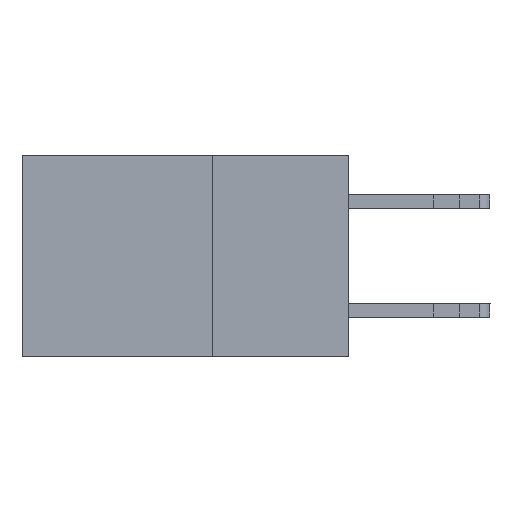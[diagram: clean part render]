
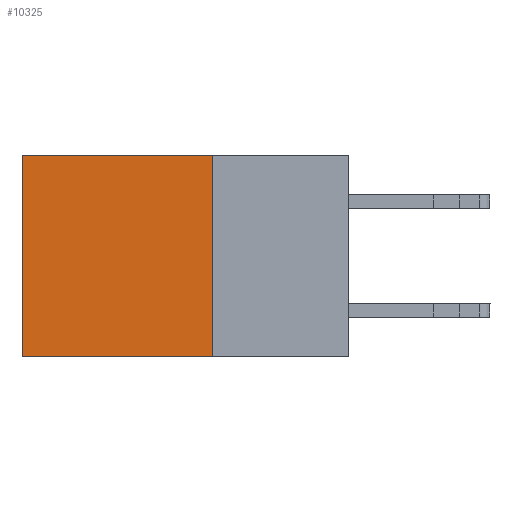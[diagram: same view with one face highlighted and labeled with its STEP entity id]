
A CAD part, left-side view. The second image highlights one B-rep face of the part: STEP entity #10325.
In plain terms, the highlighted planar face has unit normal (-1, 0, 0).
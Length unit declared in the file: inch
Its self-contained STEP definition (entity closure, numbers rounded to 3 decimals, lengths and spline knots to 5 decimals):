
#397 = DIRECTION ( 'NONE',  ( 0., 1., 0. ) ) ;
#1398 = ORIENTED_EDGE ( 'NONE', *, *, #6215, .T. ) ;
#1501 = VERTEX_POINT ( 'NONE', #11017 ) ;
#3024 = VERTEX_POINT ( 'NONE', #6247 ) ;
#3731 = EDGE_CURVE ( 'NONE', #3024, #3806, #9704, .T. ) ;
#3806 = VERTEX_POINT ( 'NONE', #9852 ) ;
#4401 = DIRECTION ( 'NONE',  ( 1., 0., 0. ) ) ;
#4995 = DIRECTION ( 'NONE',  ( 0., 0., -1. ) ) ;
#5463 = ORIENTED_EDGE ( 'NONE', *, *, #3731, .T. ) ;
#5801 = EDGE_LOOP ( 'NONE', ( #1398, #9875, #6240, #5463 ) ) ;
#6215 = EDGE_CURVE ( 'NONE', #3806, #8680, #7964, .T. ) ;
#6240 = ORIENTED_EDGE ( 'NONE', *, *, #12989, .F. ) ;
#6247 = CARTESIAN_POINT ( 'NONE',  ( 0.2615, 0.25, 0. ) ) ;
#7080 = VECTOR ( 'NONE', #4995, 39.37008 ) ;
#7309 = DIRECTION ( 'NONE',  ( 0., 0., -1. ) ) ;
#7462 = CARTESIAN_POINT ( 'NONE',  ( 0.2615, 0.25, -0.37 ) ) ;
#7715 = CARTESIAN_POINT ( 'NONE',  ( 0.2615, 0.6, -0.37 ) ) ;
#7964 = LINE ( 'NONE', #7715, #12870 ) ;
#8017 = EDGE_CURVE ( 'NONE', #1501, #8680, #9854, .T. ) ;
#8680 = VERTEX_POINT ( 'NONE', #9933 ) ;
#9081 = CARTESIAN_POINT ( 'NONE',  ( 0.2615, 0.25, -0.37 ) ) ;
#9363 = FACE_OUTER_BOUND ( 'NONE', #5801, .T. ) ;
#9546 = VECTOR ( 'NONE', #397, 39.37008 ) ;
#9704 = LINE ( 'NONE', #10245, #12301 ) ;
#9729 = CARTESIAN_POINT ( 'NONE',  ( 0.2615, 0.25, -0.37 ) ) ;
#9852 = CARTESIAN_POINT ( 'NONE',  ( 0.2615, 0.6, 0. ) ) ;
#9854 = LINE ( 'NONE', #9729, #9546 ) ;
#9875 = ORIENTED_EDGE ( 'NONE', *, *, #8017, .F. ) ;
#9933 = CARTESIAN_POINT ( 'NONE',  ( 0.2615, 0.6, -0.37 ) ) ;
#10043 = LINE ( 'NONE', #9081, #7080 ) ;
#10245 = CARTESIAN_POINT ( 'NONE',  ( 0.2615, 0.25, 0. ) ) ;
#10325 = ADVANCED_FACE ( 'NONE', ( #9363 ), #10456, .F. ) ;
#10456 = PLANE ( 'NONE',  #11422 ) ;
#10801 = DIRECTION ( 'NONE',  ( 0., 1., 0. ) ) ;
#11017 = CARTESIAN_POINT ( 'NONE',  ( 0.2615, 0.25, -0.37 ) ) ;
#11422 = AXIS2_PLACEMENT_3D ( 'NONE', #7462, #4401, #11449 ) ;
#11449 = DIRECTION ( 'NONE',  ( 0., 0., -1. ) ) ;
#12301 = VECTOR ( 'NONE', #10801, 39.37008 ) ;
#12870 = VECTOR ( 'NONE', #7309, 39.37008 ) ;
#12989 = EDGE_CURVE ( 'NONE', #3024, #1501, #10043, .T. ) ;
